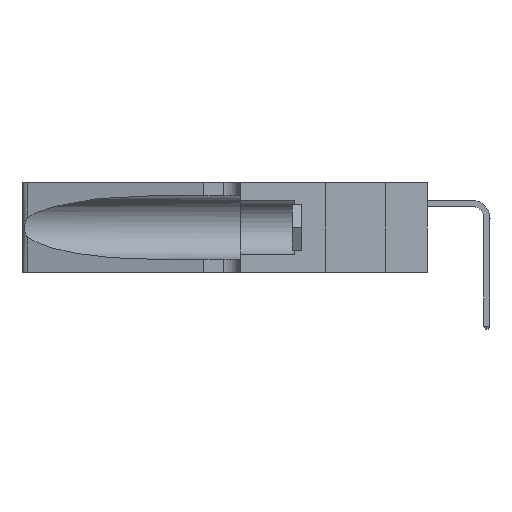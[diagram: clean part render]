
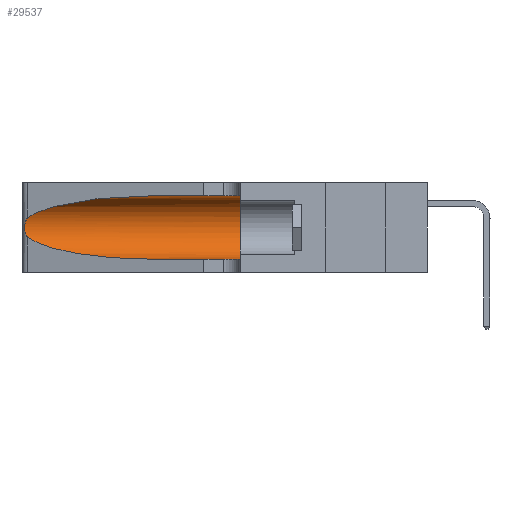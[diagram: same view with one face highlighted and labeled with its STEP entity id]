
A CAD part, left-side view. The second image highlights one B-rep face of the part: STEP entity #29537.
In plain terms, the highlighted cylindrical face has radius 3.308 mm (diameter 6.617 mm), a partial arc.
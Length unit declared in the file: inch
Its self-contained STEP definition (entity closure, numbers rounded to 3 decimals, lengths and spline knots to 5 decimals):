
#227 = ORIENTED_EDGE ( 'NONE', *, *, #36518, .F. ) ;
#1343 = CARTESIAN_POINT ( 'NONE',  ( 0.1305, 1.61858, 0.05475 ) ) ;
#2669 = CARTESIAN_POINT ( 'NONE',  ( 0.1305, 0.35, 0.05475 ) ) ;
#3190 = CARTESIAN_POINT ( 'NONE',  ( 0.25487, 1.22718, 0.14631 ) ) ;
#3788 = CARTESIAN_POINT ( 'NONE',  ( 0.1305, 1.61858, 0.185 ) ) ;
#4009 = EDGE_LOOP ( 'NONE', ( #30582, #9433, #7923, #8122, #42656, #227 ) ) ;
#4955 = DIRECTION ( 'NONE',  ( 0., 1., 0. ) ) ;
#5053 = DIRECTION ( 'NONE',  ( 0., -1., 0. ) ) ;
#5731 = VECTOR ( 'NONE', #36226, 39.37008 ) ;
#6737 = CARTESIAN_POINT ( 'NONE',  ( 0.25639, 1.23184, 0.21858 ) ) ;
#6836 = CARTESIAN_POINT ( 'NONE',  ( 0.1305, 1.61858, 0.31525 ) ) ;
#7923 = ORIENTED_EDGE ( 'NONE', *, *, #24406, .T. ) ;
#8122 = ORIENTED_EDGE ( 'NONE', *, *, #47248, .T. ) ;
#9433 = ORIENTED_EDGE ( 'NONE', *, *, #21765, .T. ) ;
#10371 = CARTESIAN_POINT ( 'NONE',  ( 0.25854, 1.2359, 0.20912 ) ) ;
#11215 = AXIS2_PLACEMENT_3D ( 'NONE', #3788, #44250, #18390 ) ;
#12000 =( BOUNDED_CURVE ( )  B_SPLINE_CURVE ( 3, ( #39764, #14044, #21474, #47132 ),
 .UNSPECIFIED., .F., .F. ) 
 B_SPLINE_CURVE_WITH_KNOTS ( ( 4, 4 ),
 ( 3.44316, 4.71239 ),
 .UNSPECIFIED. ) 
 CURVE ( )  GEOMETRIC_REPRESENTATION_ITEM ( )  RATIONAL_B_SPLINE_CURVE ( ( 1., 0.87, 0.87, 1. ) ) 
 REPRESENTATION_ITEM ( '' )  );
#12589 = CARTESIAN_POINT ( 'NONE',  ( 0.1305, 0.72297, 0.31525 ) ) ;
#13133 = VERTEX_POINT ( 'NONE', #34479 ) ;
#14044 = CARTESIAN_POINT ( 'NONE',  ( 0.2373, 1.15595, 0.08982 ) ) ;
#14083 = CARTESIAN_POINT ( 'NONE',  ( 0.26075, 1.23896, 0.19203 ) ) ;
#14907 = VERTEX_POINT ( 'NONE', #40921 ) ;
#15477 = LINE ( 'NONE', #6836, #5731 ) ;
#16130 = LINE ( 'NONE', #1343, #38683 ) ;
#16902 = CIRCLE ( 'NONE', #24293, 0.13025 ) ;
#16968 = CARTESIAN_POINT ( 'NONE',  ( 0.1305, 0.72297, 0.31525 ) ) ;
#17711 = VERTEX_POINT ( 'NONE', #12589 ) ;
#17790 = CARTESIAN_POINT ( 'NONE',  ( 0.26017, 1.23833, 0.17102 ) ) ;
#18390 = DIRECTION ( 'NONE',  ( 0., 0., -1. ) ) ;
#20688 = CARTESIAN_POINT ( 'NONE',  ( 0.2373, 1.15595, 0.28018 ) ) ;
#21336 = CARTESIAN_POINT ( 'NONE',  ( 0.25487, 1.22718, 0.22369 ) ) ;
#21474 = CARTESIAN_POINT ( 'NONE',  ( 0.18966, 0.96281, 0.05475 ) ) ;
#21497 = CARTESIAN_POINT ( 'NONE',  ( 0.25789, 1.23486, 0.15765 ) ) ;
#21765 = EDGE_CURVE ( 'NONE', #14907, #13133, #28495, .T. ) ;
#24293 = AXIS2_PLACEMENT_3D ( 'NONE', #26931, #4955, #30640 ) ;
#24406 = EDGE_CURVE ( 'NONE', #13133, #43820, #12000, .T. ) ;
#25180 = CARTESIAN_POINT ( 'NONE',  ( 0.25555, 1.22993, 0.14849 ) ) ;
#26296 = VERTEX_POINT ( 'NONE', #2669 ) ;
#26931 = CARTESIAN_POINT ( 'NONE',  ( 0.1305, 0.35, 0.185 ) ) ;
#28495 = B_SPLINE_CURVE_WITH_KNOTS ( 'NONE', 3,
 ( #21336, #39635, #6737, #32405, #10371, #36120, #14083, #39792, #17790, #43484, #21497, #47164, #25180, #3190 ),
 .UNSPECIFIED., .F., .F.,
 ( 4, 2, 2, 2, 2, 2, 4 ),
 ( 0., 0.00027, 0.00053, 0.00107, 0.0016, 0.00187, 0.00214 ),
 .UNSPECIFIED. ) ;
#29537 = ADVANCED_FACE ( 'NONE', ( #41119 ), #39984, .F. ) ;
#30582 = ORIENTED_EDGE ( 'NONE', *, *, #39446, .T. ) ;
#30640 = DIRECTION ( 'NONE',  ( 0., 0., 1. ) ) ;
#32405 = CARTESIAN_POINT ( 'NONE',  ( 0.25787, 1.23484, 0.2124 ) ) ;
#33221 = CARTESIAN_POINT ( 'NONE',  ( 0.1305, 0.72297, 0.05475 ) ) ;
#34479 = CARTESIAN_POINT ( 'NONE',  ( 0.25487, 1.22718, 0.14631 ) ) ;
#36120 = CARTESIAN_POINT ( 'NONE',  ( 0.26018, 1.23835, 0.19895 ) ) ;
#36226 = DIRECTION ( 'NONE',  ( 0., -1., 0. ) ) ;
#36518 = EDGE_CURVE ( 'NONE', #17711, #46525, #15477, .T. ) ;
#38683 = VECTOR ( 'NONE', #5053, 39.37008 ) ;
#39249 = EDGE_CURVE ( 'NONE', #46525, #26296, #16902, .T. ) ;
#39446 = EDGE_CURVE ( 'NONE', #17711, #14907, #45349, .T. ) ;
#39635 = CARTESIAN_POINT ( 'NONE',  ( 0.25555, 1.22994, 0.2215 ) ) ;
#39764 = CARTESIAN_POINT ( 'NONE',  ( 0.25487, 1.22718, 0.14631 ) ) ;
#39792 = CARTESIAN_POINT ( 'NONE',  ( 0.26075, 1.23896, 0.178 ) ) ;
#39984 = CYLINDRICAL_SURFACE ( 'NONE', #11215, 0.13025 ) ;
#40921 = CARTESIAN_POINT ( 'NONE',  ( 0.25487, 1.22718, 0.22369 ) ) ;
#41119 = FACE_OUTER_BOUND ( 'NONE', #4009, .T. ) ;
#42656 = ORIENTED_EDGE ( 'NONE', *, *, #39249, .F. ) ;
#42659 = CARTESIAN_POINT ( 'NONE',  ( 0.18966, 0.96281, 0.31525 ) ) ;
#43484 = CARTESIAN_POINT ( 'NONE',  ( 0.25856, 1.23593, 0.16098 ) ) ;
#43820 = VERTEX_POINT ( 'NONE', #33221 ) ;
#44250 = DIRECTION ( 'NONE',  ( 0., -1., 0. ) ) ;
#44941 = CARTESIAN_POINT ( 'NONE',  ( 0.1305, 0.35, 0.31525 ) ) ;
#45349 =( BOUNDED_CURVE ( )  B_SPLINE_CURVE ( 3, ( #16968, #42659, #20688, #46360 ),
 .UNSPECIFIED., .F., .T. ) 
 B_SPLINE_CURVE_WITH_KNOTS ( ( 4, 4 ),
 ( 1.5708, 2.84003 ),
 .UNSPECIFIED. ) 
 CURVE ( )  GEOMETRIC_REPRESENTATION_ITEM ( )  RATIONAL_B_SPLINE_CURVE ( ( 1., 0.87, 0.87, 1. ) ) 
 REPRESENTATION_ITEM ( '' )  );
#46360 = CARTESIAN_POINT ( 'NONE',  ( 0.25487, 1.22718, 0.22369 ) ) ;
#46525 = VERTEX_POINT ( 'NONE', #44941 ) ;
#47132 = CARTESIAN_POINT ( 'NONE',  ( 0.1305, 0.72297, 0.05475 ) ) ;
#47164 = CARTESIAN_POINT ( 'NONE',  ( 0.25639, 1.23186, 0.15144 ) ) ;
#47248 = EDGE_CURVE ( 'NONE', #43820, #26296, #16130, .T. ) ;
